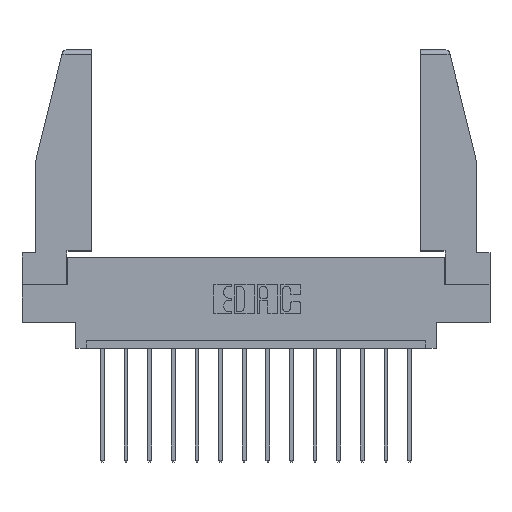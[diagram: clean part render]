
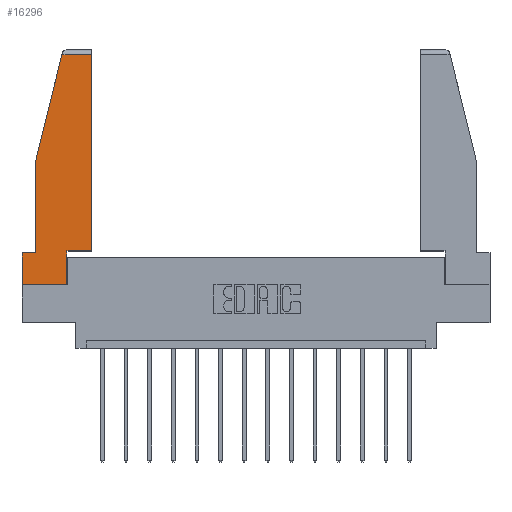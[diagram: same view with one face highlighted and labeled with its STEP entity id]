
A CAD part, top view. The second image highlights one B-rep face of the part: STEP entity #16296.
In plain terms, the highlighted planar face has unit normal (0, 0, 1).
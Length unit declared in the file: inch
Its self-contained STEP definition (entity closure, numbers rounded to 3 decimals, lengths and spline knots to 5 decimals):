
#269 = DIRECTION ( 'NONE',  ( -1., 0., 0. ) ) ;
#332 = ORIENTED_EDGE ( 'NONE', *, *, #15165, .T. ) ;
#618 = LINE ( 'NONE', #5864, #2648 ) ;
#651 = CARTESIAN_POINT ( 'NONE',  ( 0., 0., 0. ) ) ;
#857 = EDGE_CURVE ( 'NONE', #12611, #4942, #15717, .T. ) ;
#894 = ORIENTED_EDGE ( 'NONE', *, *, #11865, .T. ) ;
#999 = VERTEX_POINT ( 'NONE', #14521 ) ;
#1189 = EDGE_CURVE ( 'NONE', #13253, #5135, #618, .T. ) ;
#1214 = VERTEX_POINT ( 'NONE', #3411 ) ;
#1251 = ORIENTED_EDGE ( 'NONE', *, *, #11095, .T. ) ;
#1322 = VERTEX_POINT ( 'NONE', #9969 ) ;
#1354 = ORIENTED_EDGE ( 'NONE', *, *, #10553, .T. ) ;
#2211 = VECTOR ( 'NONE', #14566, 39.37008 ) ;
#2234 = AXIS2_PLACEMENT_3D ( 'NONE', #12403, #11006, #13522 ) ;
#2255 = ORIENTED_EDGE ( 'NONE', *, *, #1189, .T. ) ;
#2539 = ORIENTED_EDGE ( 'NONE', *, *, #857, .T. ) ;
#2648 = VECTOR ( 'NONE', #12348, 39.37008 ) ;
#3296 = CARTESIAN_POINT ( 'NONE',  ( 0.2636, 1.52, 0. ) ) ;
#3411 = CARTESIAN_POINT ( 'NONE',  ( 0.461, 0.223, 0. ) ) ;
#3519 = CARTESIAN_POINT ( 'NONE',  ( 0.086, 0.21, 0. ) ) ;
#3585 = VERTEX_POINT ( 'NONE', #3519 ) ;
#3677 = LINE ( 'NONE', #8400, #16158 ) ;
#4196 = LINE ( 'NONE', #13336, #2211 ) ;
#4551 = DIRECTION ( 'NONE',  ( 0., 1., 0. ) ) ;
#4858 = VECTOR ( 'NONE', #269, 39.37008 ) ;
#4942 = VERTEX_POINT ( 'NONE', #3296 ) ;
#5135 = VERTEX_POINT ( 'NONE', #13351 ) ;
#5299 = CARTESIAN_POINT ( 'NONE',  ( 0., 1.52, 0. ) ) ;
#5588 = VECTOR ( 'NONE', #14976, 39.37008 ) ;
#5808 = DIRECTION ( 'NONE',  ( 0., -1., 0. ) ) ;
#5864 = CARTESIAN_POINT ( 'NONE',  ( 0., 0., 0. ) ) ;
#6353 = EDGE_LOOP ( 'NONE', ( #1251, #2539, #332, #16087, #894, #16211, #2255, #7805, #1354 ) ) ;
#6444 = VECTOR ( 'NONE', #15374, 39.37008 ) ;
#6484 = VECTOR ( 'NONE', #15861, 39.37008 ) ;
#6927 = VERTEX_POINT ( 'NONE', #11824 ) ;
#6994 = CARTESIAN_POINT ( 'NONE',  ( 0., 0.21, 0. ) ) ;
#7805 = ORIENTED_EDGE ( 'NONE', *, *, #9537, .T. ) ;
#8400 = CARTESIAN_POINT ( 'NONE',  ( 0.086, 0.8, 0. ) ) ;
#8700 = EDGE_CURVE ( 'NONE', #6927, #3585, #3677, .T. ) ;
#9371 = VECTOR ( 'NONE', #4551, 39.37008 ) ;
#9537 = EDGE_CURVE ( 'NONE', #5135, #999, #16126, .T. ) ;
#9969 = CARTESIAN_POINT ( 'NONE',  ( 0., 0.21, 0. ) ) ;
#10359 = CARTESIAN_POINT ( 'NONE',  ( 0.297, 0., 0. ) ) ;
#10553 = EDGE_CURVE ( 'NONE', #999, #1214, #12469, .T. ) ;
#10689 = FACE_OUTER_BOUND ( 'NONE', #6353, .T. ) ;
#10891 = CARTESIAN_POINT ( 'NONE',  ( 0.297, 0.223, 0. ) ) ;
#11006 = DIRECTION ( 'NONE',  ( 0., 0., 1. ) ) ;
#11095 = EDGE_CURVE ( 'NONE', #1214, #12611, #14331, .T. ) ;
#11142 = CARTESIAN_POINT ( 'NONE',  ( 0.461, 0.223, 0. ) ) ;
#11336 = EDGE_CURVE ( 'NONE', #1322, #13253, #11876, .T. ) ;
#11824 = CARTESIAN_POINT ( 'NONE',  ( 0.086, 0.8, 0. ) ) ;
#11865 = EDGE_CURVE ( 'NONE', #3585, #1322, #4196, .T. ) ;
#11876 = LINE ( 'NONE', #6994, #16106 ) ;
#12049 = CARTESIAN_POINT ( 'NONE',  ( 0.271, 1.55, 0. ) ) ;
#12345 = PLANE ( 'NONE',  #2234 ) ;
#12348 = DIRECTION ( 'NONE',  ( 1., 0., 0. ) ) ;
#12403 = CARTESIAN_POINT ( 'NONE',  ( 0., 0., 0. ) ) ;
#12469 = LINE ( 'NONE', #10891, #5588 ) ;
#12611 = VERTEX_POINT ( 'NONE', #13168 ) ;
#13168 = CARTESIAN_POINT ( 'NONE',  ( 0.461, 1.52, 0. ) ) ;
#13253 = VERTEX_POINT ( 'NONE', #651 ) ;
#13324 = LINE ( 'NONE', #12049, #6484 ) ;
#13336 = CARTESIAN_POINT ( 'NONE',  ( 0., 0.21, 0. ) ) ;
#13351 = CARTESIAN_POINT ( 'NONE',  ( 0.297, 0., 0. ) ) ;
#13522 = DIRECTION ( 'NONE',  ( 1., 0., 0. ) ) ;
#14331 = LINE ( 'NONE', #11142, #9371 ) ;
#14521 = CARTESIAN_POINT ( 'NONE',  ( 0.297, 0.223, 0. ) ) ;
#14566 = DIRECTION ( 'NONE',  ( -1., 0., 0. ) ) ;
#14758 = DIRECTION ( 'NONE',  ( 0., -1., 0. ) ) ;
#14976 = DIRECTION ( 'NONE',  ( 1., 0., 0. ) ) ;
#15165 = EDGE_CURVE ( 'NONE', #4942, #6927, #13324, .T. ) ;
#15374 = DIRECTION ( 'NONE',  ( 0., 1., 0. ) ) ;
#15717 = LINE ( 'NONE', #5299, #4858 ) ;
#15861 = DIRECTION ( 'NONE',  ( -0.239, -0.971, 0. ) ) ;
#16087 = ORIENTED_EDGE ( 'NONE', *, *, #8700, .T. ) ;
#16106 = VECTOR ( 'NONE', #14758, 39.37008 ) ;
#16126 = LINE ( 'NONE', #10359, #6444 ) ;
#16158 = VECTOR ( 'NONE', #5808, 39.37008 ) ;
#16211 = ORIENTED_EDGE ( 'NONE', *, *, #11336, .T. ) ;
#16296 = ADVANCED_FACE ( 'NONE', ( #10689 ), #12345, .T. ) ;
